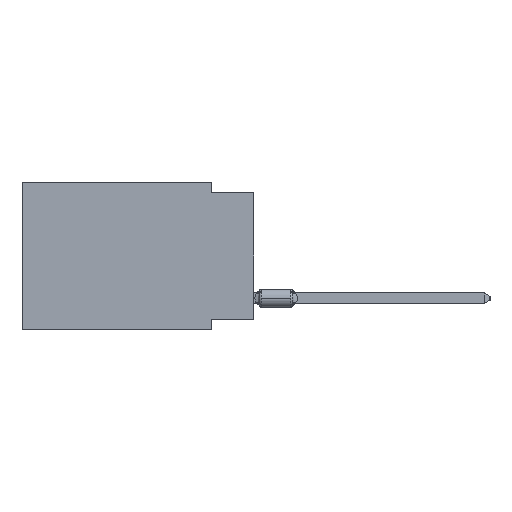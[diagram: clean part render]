
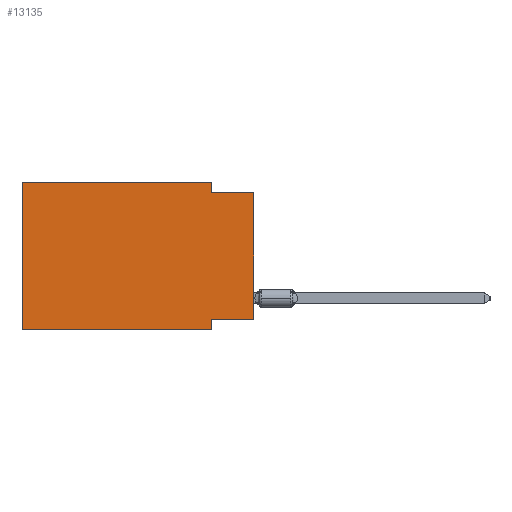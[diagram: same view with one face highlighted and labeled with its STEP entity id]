
A CAD part, left-side view. The second image highlights one B-rep face of the part: STEP entity #13135.
In plain terms, the highlighted planar face has unit normal (-1, 0, 0).
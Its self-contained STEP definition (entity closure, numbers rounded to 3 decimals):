
#129 = VECTOR ( 'NONE', #30909, 1000. ) ;
#2272 = CARTESIAN_POINT ( 'NONE',  ( 0., 0., -0.635 ) ) ;
#4424 = LINE ( 'NONE', #31447, #36577 ) ;
#4854 = LINE ( 'NONE', #31871, #26718 ) ;
#5440 = CARTESIAN_POINT ( 'NONE',  ( 0., 2.54, 0. ) ) ;
#5486 = ORIENTED_EDGE ( 'NONE', *, *, #21735, .F. ) ;
#6185 = VERTEX_POINT ( 'NONE', #5440 ) ;
#6249 = VECTOR ( 'NONE', #22774, 1000. ) ;
#6331 = VERTEX_POINT ( 'NONE', #32263 ) ;
#7723 = EDGE_CURVE ( 'NONE', #6331, #21243, #31288, .T. ) ;
#9506 = CARTESIAN_POINT ( 'NONE',  ( 0., 2.54, -0.635 ) ) ;
#10289 = VERTEX_POINT ( 'NONE', #15019 ) ;
#10454 = LINE ( 'NONE', #19126, #129 ) ;
#11563 = DIRECTION ( 'NONE',  ( 0., 0., -1. ) ) ;
#11622 = ORIENTED_EDGE ( 'NONE', *, *, #28256, .T. ) ;
#11946 = ORIENTED_EDGE ( 'NONE', *, *, #35318, .F. ) ;
#12029 = VECTOR ( 'NONE', #26545, 1000. ) ;
#12237 = ORIENTED_EDGE ( 'NONE', *, *, #33267, .F. ) ;
#12265 = DIRECTION ( 'NONE',  ( 0., 0., -1. ) ) ;
#13135 = ADVANCED_FACE ( 'NONE', ( #16811 ), #34561, .F. ) ;
#13537 = VERTEX_POINT ( 'NONE', #2272 ) ;
#13575 = CARTESIAN_POINT ( 'NONE',  ( 0., 13.97, 0. ) ) ;
#14445 = LINE ( 'NONE', #32400, #28796 ) ;
#15019 = CARTESIAN_POINT ( 'NONE',  ( 0., 13.97, 0. ) ) ;
#16610 = CARTESIAN_POINT ( 'NONE',  ( 0., 13.97, 0. ) ) ;
#16811 = FACE_OUTER_BOUND ( 'NONE', #28977, .T. ) ;
#19126 = CARTESIAN_POINT ( 'NONE',  ( 0., 0., -0.635 ) ) ;
#19291 = DIRECTION ( 'NONE',  ( 0., 0., 1. ) ) ;
#19318 = CARTESIAN_POINT ( 'NONE',  ( 0., 13.97, -8.89 ) ) ;
#19707 = DIRECTION ( 'NONE',  ( 0., 1., 0. ) ) ;
#21243 = VERTEX_POINT ( 'NONE', #30569 ) ;
#21735 = EDGE_CURVE ( 'NONE', #10289, #6185, #29629, .T. ) ;
#22774 = DIRECTION ( 'NONE',  ( 0., -1., 0. ) ) ;
#23292 = EDGE_CURVE ( 'NONE', #6185, #33101, #14445, .T. ) ;
#25310 = DIRECTION ( 'NONE',  ( 1., 0., 0. ) ) ;
#25478 = VERTEX_POINT ( 'NONE', #28033 ) ;
#26545 = DIRECTION ( 'NONE',  ( 0., -1., 0. ) ) ;
#26718 = VECTOR ( 'NONE', #19707, 1000. ) ;
#28033 = CARTESIAN_POINT ( 'NONE',  ( 0., 2.54, -8.255 ) ) ;
#28063 = LINE ( 'NONE', #13575, #31623 ) ;
#28256 = EDGE_CURVE ( 'NONE', #30450, #13537, #4424, .T. ) ;
#28380 = DIRECTION ( 'NONE',  ( 0., 0., -1. ) ) ;
#28796 = VECTOR ( 'NONE', #11563, 1000. ) ;
#28977 = EDGE_LOOP ( 'NONE', ( #11622, #12237, #30734, #5486, #29769, #32349, #30110, #11946 ) ) ;
#29397 = CARTESIAN_POINT ( 'NONE',  ( 0., 0., -8.255 ) ) ;
#29629 = LINE ( 'NONE', #32364, #12029 ) ;
#29769 = ORIENTED_EDGE ( 'NONE', *, *, #34010, .F. ) ;
#30110 = ORIENTED_EDGE ( 'NONE', *, *, #36400, .F. ) ;
#30205 = CARTESIAN_POINT ( 'NONE',  ( 0., 2.54, -8.89 ) ) ;
#30409 = LINE ( 'NONE', #30205, #31754 ) ;
#30450 = VERTEX_POINT ( 'NONE', #29397 ) ;
#30569 = CARTESIAN_POINT ( 'NONE',  ( 0., 2.54, -8.89 ) ) ;
#30734 = ORIENTED_EDGE ( 'NONE', *, *, #23292, .F. ) ;
#30909 = DIRECTION ( 'NONE',  ( 0., -1., 0. ) ) ;
#31288 = LINE ( 'NONE', #19318, #6249 ) ;
#31447 = CARTESIAN_POINT ( 'NONE',  ( 0., 0., 0. ) ) ;
#31623 = VECTOR ( 'NONE', #37336, 1000. ) ;
#31754 = VECTOR ( 'NONE', #12265, 1000. ) ;
#31871 = CARTESIAN_POINT ( 'NONE',  ( 0., 0., -8.255 ) ) ;
#32263 = CARTESIAN_POINT ( 'NONE',  ( 0., 13.97, -8.89 ) ) ;
#32349 = ORIENTED_EDGE ( 'NONE', *, *, #7723, .T. ) ;
#32364 = CARTESIAN_POINT ( 'NONE',  ( 0., 13.97, 0. ) ) ;
#32400 = CARTESIAN_POINT ( 'NONE',  ( 0., 2.54, 0. ) ) ;
#33101 = VERTEX_POINT ( 'NONE', #9506 ) ;
#33267 = EDGE_CURVE ( 'NONE', #33101, #13537, #10454, .T. ) ;
#33470 = AXIS2_PLACEMENT_3D ( 'NONE', #16610, #25310, #28380 ) ;
#34010 = EDGE_CURVE ( 'NONE', #6331, #10289, #28063, .T. ) ;
#34561 = PLANE ( 'NONE',  #33470 ) ;
#35318 = EDGE_CURVE ( 'NONE', #30450, #25478, #4854, .T. ) ;
#36400 = EDGE_CURVE ( 'NONE', #25478, #21243, #30409, .T. ) ;
#36577 = VECTOR ( 'NONE', #19291, 1000. ) ;
#37336 = DIRECTION ( 'NONE',  ( 0., 0., 1. ) ) ;
